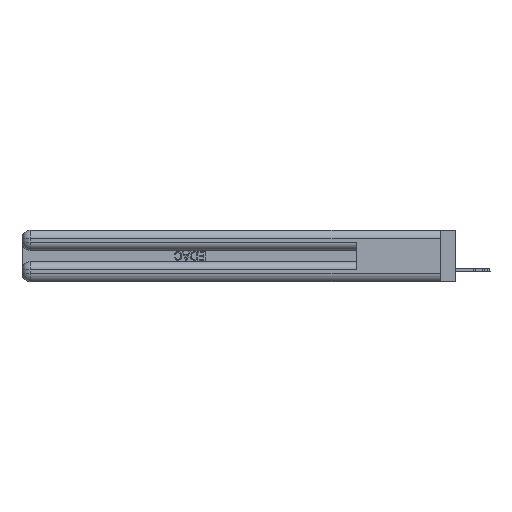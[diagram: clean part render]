
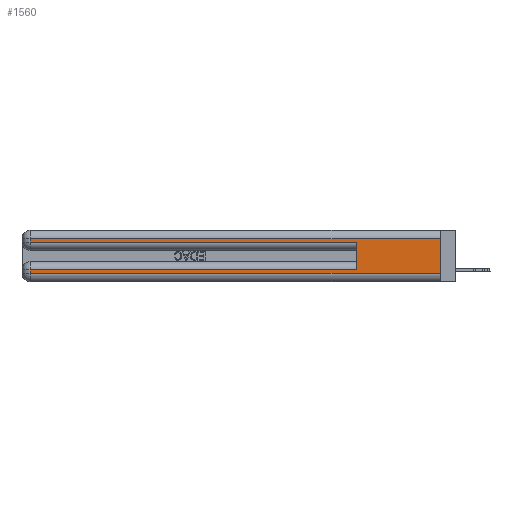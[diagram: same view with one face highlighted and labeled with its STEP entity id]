
A CAD part, left-side view. The second image highlights one B-rep face of the part: STEP entity #1560.
In plain terms, the highlighted planar face has unit normal (-1, 0, 0).
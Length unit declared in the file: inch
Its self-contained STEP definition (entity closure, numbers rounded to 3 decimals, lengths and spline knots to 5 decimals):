
#1247 = EDGE_CURVE ( 'NONE', #25061, #28930, #36294, .T. ) ;
#1560 = ADVANCED_FACE ( 'NONE', ( #17966 ), #31816, .F. ) ;
#3512 = DIRECTION ( 'NONE',  ( 0., 1., 0. ) ) ;
#4343 = DIRECTION ( 'NONE',  ( 0., 0., -1. ) ) ;
#4501 = ORIENTED_EDGE ( 'NONE', *, *, #34804, .T. ) ;
#4692 = ORIENTED_EDGE ( 'NONE', *, *, #40788, .T. ) ;
#5612 = DIRECTION ( 'NONE',  ( 0., 0., -1. ) ) ;
#7073 = CARTESIAN_POINT ( 'NONE',  ( 0., 2.94, 0.085 ) ) ;
#7227 = CARTESIAN_POINT ( 'NONE',  ( 0., 0.6, 0.145 ) ) ;
#8174 = VERTEX_POINT ( 'NONE', #7073 ) ;
#8741 = VERTEX_POINT ( 'NONE', #18650 ) ;
#9002 = DIRECTION ( 'NONE',  ( 0., -1., 0. ) ) ;
#9123 = DIRECTION ( 'NONE',  ( 0., 1., 0. ) ) ;
#10262 = ORIENTED_EDGE ( 'NONE', *, *, #35825, .T. ) ;
#10854 = DIRECTION ( 'NONE',  ( 1., 0., 0. ) ) ;
#11861 = VECTOR ( 'NONE', #5612, 39.37008 ) ;
#12254 = DIRECTION ( 'NONE',  ( 0., 0., 1. ) ) ;
#13073 = LINE ( 'NONE', #42663, #11861 ) ;
#14549 = CARTESIAN_POINT ( 'NONE',  ( 0., 0., 0.06 ) ) ;
#15033 = LINE ( 'NONE', #30577, #42752 ) ;
#15606 = VECTOR ( 'NONE', #36353, 39.37008 ) ;
#16564 = VECTOR ( 'NONE', #9123, 39.37008 ) ;
#17028 = ORIENTED_EDGE ( 'NONE', *, *, #1247, .F. ) ;
#17966 = FACE_OUTER_BOUND ( 'NONE', #34954, .T. ) ;
#18195 = ORIENTED_EDGE ( 'NONE', *, *, #43746, .T. ) ;
#18650 = CARTESIAN_POINT ( 'NONE',  ( 0., 2.94, 0.06 ) ) ;
#19067 = DIRECTION ( 'NONE',  ( 0., 0., -1. ) ) ;
#19824 = CARTESIAN_POINT ( 'NONE',  ( 0., 0., 0.285 ) ) ;
#20001 = VECTOR ( 'NONE', #9002, 39.37008 ) ;
#21002 = VERTEX_POINT ( 'NONE', #34797 ) ;
#21104 = EDGE_CURVE ( 'NONE', #44836, #53091, #30708, .T. ) ;
#21802 = ORIENTED_EDGE ( 'NONE', *, *, #21104, .F. ) ;
#23059 = CARTESIAN_POINT ( 'NONE',  ( 0., 0., 0.37 ) ) ;
#25061 = VERTEX_POINT ( 'NONE', #48734 ) ;
#25560 = ORIENTED_EDGE ( 'NONE', *, *, #48681, .T. ) ;
#26483 = CARTESIAN_POINT ( 'NONE',  ( 0., 2.94, 0.31 ) ) ;
#28594 = CARTESIAN_POINT ( 'NONE',  ( 0., 0., 0.37 ) ) ;
#28930 = VERTEX_POINT ( 'NONE', #14549 ) ;
#29266 = CARTESIAN_POINT ( 'NONE',  ( 0., 0., 0.06 ) ) ;
#30399 = VERTEX_POINT ( 'NONE', #26483 ) ;
#30577 = CARTESIAN_POINT ( 'NONE',  ( 0., 2.94, 0.37 ) ) ;
#30708 = LINE ( 'NONE', #7227, #32743 ) ;
#31816 = PLANE ( 'NONE',  #40467 ) ;
#32743 = VECTOR ( 'NONE', #12254, 39.37008 ) ;
#33740 = VECTOR ( 'NONE', #3512, 39.37008 ) ;
#33951 = CARTESIAN_POINT ( 'NONE',  ( 0., 0.6, 0.285 ) ) ;
#34750 = DIRECTION ( 'NONE',  ( 0., 0., -1. ) ) ;
#34797 = CARTESIAN_POINT ( 'NONE',  ( 0., 2.94, 0.285 ) ) ;
#34804 = EDGE_CURVE ( 'NONE', #30399, #21002, #15033, .T. ) ;
#34903 = VECTOR ( 'NONE', #4343, 39.37008 ) ;
#34954 = EDGE_LOOP ( 'NONE', ( #17028, #25560, #4501, #18195, #21802, #4692, #39864, #10262 ) ) ;
#35662 = CARTESIAN_POINT ( 'NONE',  ( 0., 0.6, 0.085 ) ) ;
#35825 = EDGE_CURVE ( 'NONE', #8741, #28930, #41983, .T. ) ;
#36294 = LINE ( 'NONE', #28594, #34903 ) ;
#36353 = DIRECTION ( 'NONE',  ( 0., -1., 0. ) ) ;
#38036 = CARTESIAN_POINT ( 'NONE',  ( 0., 0., 0.085 ) ) ;
#39864 = ORIENTED_EDGE ( 'NONE', *, *, #42627, .T. ) ;
#40182 = LINE ( 'NONE', #19824, #15606 ) ;
#40467 = AXIS2_PLACEMENT_3D ( 'NONE', #23059, #10854, #19067 ) ;
#40550 = LINE ( 'NONE', #38036, #16564 ) ;
#40788 = EDGE_CURVE ( 'NONE', #44836, #8174, #40550, .T. ) ;
#41983 = LINE ( 'NONE', #29266, #20001 ) ;
#42627 = EDGE_CURVE ( 'NONE', #8174, #8741, #13073, .T. ) ;
#42663 = CARTESIAN_POINT ( 'NONE',  ( 0., 2.94, 0.37 ) ) ;
#42752 = VECTOR ( 'NONE', #34750, 39.37008 ) ;
#42823 = LINE ( 'NONE', #48514, #33740 ) ;
#43746 = EDGE_CURVE ( 'NONE', #21002, #53091, #40182, .T. ) ;
#44836 = VERTEX_POINT ( 'NONE', #35662 ) ;
#48514 = CARTESIAN_POINT ( 'NONE',  ( 0., 0., 0.31 ) ) ;
#48681 = EDGE_CURVE ( 'NONE', #25061, #30399, #42823, .T. ) ;
#48734 = CARTESIAN_POINT ( 'NONE',  ( 0., 0., 0.31 ) ) ;
#53091 = VERTEX_POINT ( 'NONE', #33951 ) ;
